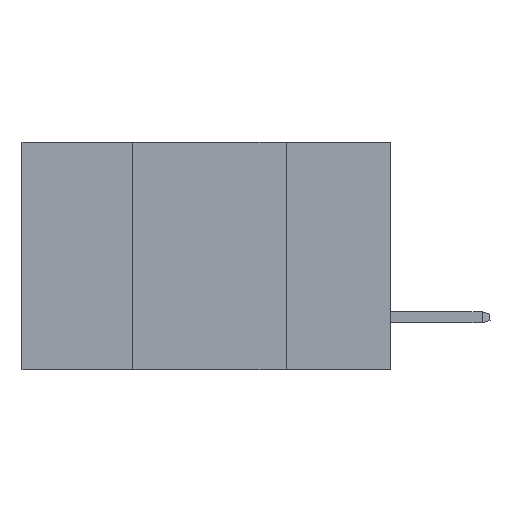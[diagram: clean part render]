
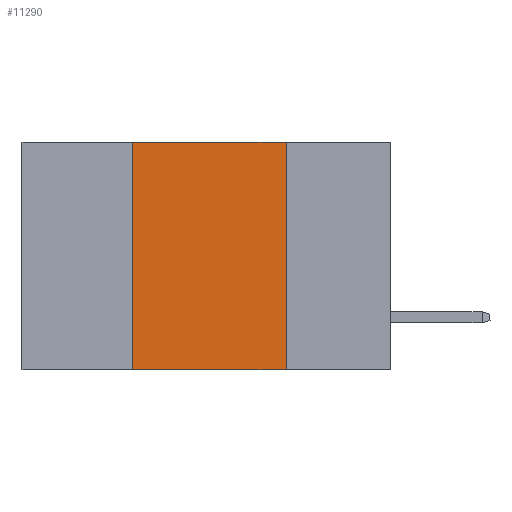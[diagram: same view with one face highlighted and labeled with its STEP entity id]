
A CAD part, left-side view. The second image highlights one B-rep face of the part: STEP entity #11290.
In plain terms, the highlighted planar face has unit normal (-1, 0, 0).
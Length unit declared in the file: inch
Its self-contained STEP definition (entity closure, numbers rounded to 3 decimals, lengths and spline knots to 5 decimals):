
#7 = DIRECTION ( 'NONE',  ( 0., 0., -1. ) ) ;
#235 = LINE ( 'NONE', #11505, #10163 ) ;
#1098 = VERTEX_POINT ( 'NONE', #3886 ) ;
#1229 = DIRECTION ( 'NONE',  ( 0., 0., 1. ) ) ;
#2556 = CARTESIAN_POINT ( 'NONE',  ( 0., 0.6, -0.37 ) ) ;
#2953 = DIRECTION ( 'NONE',  ( 1., 0., 0. ) ) ;
#2977 = VECTOR ( 'NONE', #10196, 39.37008 ) ;
#3119 = AXIS2_PLACEMENT_3D ( 'NONE', #11479, #2953, #9608 ) ;
#3287 = VERTEX_POINT ( 'NONE', #6081 ) ;
#3886 = CARTESIAN_POINT ( 'NONE',  ( 0., 0.42, 0. ) ) ;
#4242 = VECTOR ( 'NONE', #1229, 39.37008 ) ;
#5189 = EDGE_CURVE ( 'NONE', #6744, #3287, #10577, .T. ) ;
#5633 = CARTESIAN_POINT ( 'NONE',  ( 0., 0.17, 0. ) ) ;
#6081 = CARTESIAN_POINT ( 'NONE',  ( 0., 0.17, -0.37 ) ) ;
#6309 = ORIENTED_EDGE ( 'NONE', *, *, #7321, .F. ) ;
#6477 = ORIENTED_EDGE ( 'NONE', *, *, #5189, .T. ) ;
#6744 = VERTEX_POINT ( 'NONE', #7720 ) ;
#6924 = ORIENTED_EDGE ( 'NONE', *, *, #9384, .F. ) ;
#6941 = LINE ( 'NONE', #8487, #11720 ) ;
#7301 = VERTEX_POINT ( 'NONE', #5633 ) ;
#7321 = EDGE_CURVE ( 'NONE', #1098, #7301, #6941, .T. ) ;
#7720 = CARTESIAN_POINT ( 'NONE',  ( 0., 0.42, -0.37 ) ) ;
#8050 = EDGE_CURVE ( 'NONE', #6744, #1098, #11845, .T. ) ;
#8487 = CARTESIAN_POINT ( 'NONE',  ( 0., 0.6, 0. ) ) ;
#8649 = PLANE ( 'NONE',  #3119 ) ;
#9384 = EDGE_CURVE ( 'NONE', #7301, #3287, #235, .T. ) ;
#9608 = DIRECTION ( 'NONE',  ( 0., 0., -1. ) ) ;
#9620 = EDGE_LOOP ( 'NONE', ( #6924, #6309, #10357, #6477 ) ) ;
#9758 = FACE_OUTER_BOUND ( 'NONE', #9620, .T. ) ;
#9879 = CARTESIAN_POINT ( 'NONE',  ( 0., 0.42, 0. ) ) ;
#10163 = VECTOR ( 'NONE', #7, 39.37008 ) ;
#10196 = DIRECTION ( 'NONE',  ( 0., -1., 0. ) ) ;
#10357 = ORIENTED_EDGE ( 'NONE', *, *, #8050, .F. ) ;
#10410 = DIRECTION ( 'NONE',  ( 0., -1., 0. ) ) ;
#10577 = LINE ( 'NONE', #2556, #2977 ) ;
#11290 = ADVANCED_FACE ( 'NONE', ( #9758 ), #8649, .F. ) ;
#11479 = CARTESIAN_POINT ( 'NONE',  ( 0., 0.6, 0. ) ) ;
#11505 = CARTESIAN_POINT ( 'NONE',  ( 0., 0.17, 0. ) ) ;
#11720 = VECTOR ( 'NONE', #10410, 39.37008 ) ;
#11845 = LINE ( 'NONE', #9879, #4242 ) ;
